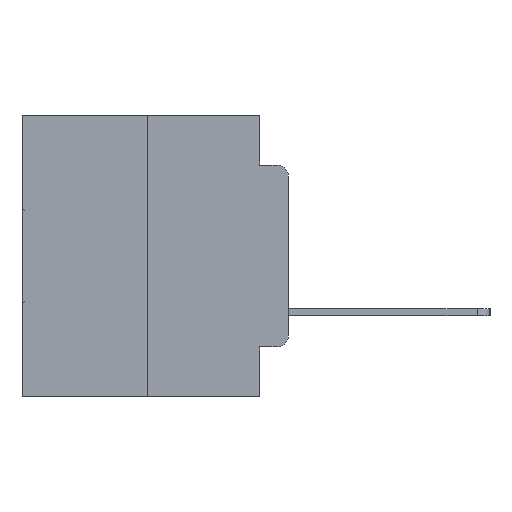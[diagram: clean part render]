
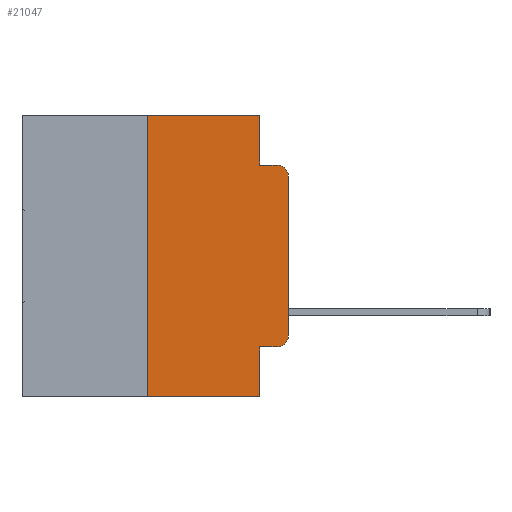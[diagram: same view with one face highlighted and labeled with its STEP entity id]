
A CAD part, left-side view. The second image highlights one B-rep face of the part: STEP entity #21047.
In plain terms, the highlighted planar face has unit normal (-1, 0, 0).
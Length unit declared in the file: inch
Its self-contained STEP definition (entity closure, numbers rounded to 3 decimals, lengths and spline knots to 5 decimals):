
#730 = LINE ( 'NONE', #3801, #25621 ) ;
#1275 = CARTESIAN_POINT ( 'NONE',  ( 0., 0.051, 0. ) ) ;
#1416 = LINE ( 'NONE', #19084, #6459 ) ;
#2512 = LINE ( 'NONE', #1275, #3318 ) ;
#3004 = AXIS2_PLACEMENT_3D ( 'NONE', #23975, #26347, #12099 ) ;
#3126 = DIRECTION ( 'NONE',  ( 0., 0., -1. ) ) ;
#3318 = VECTOR ( 'NONE', #15873, 39.37008 ) ;
#3801 = CARTESIAN_POINT ( 'NONE',  ( 0., 0.051, -0.0885 ) ) ;
#4295 = DIRECTION ( 'NONE',  ( 0., 0., 1. ) ) ;
#4416 = VECTOR ( 'NONE', #3126, 39.37008 ) ;
#5828 = VERTEX_POINT ( 'NONE', #13246 ) ;
#6107 = EDGE_LOOP ( 'NONE', ( #14253, #14192, #24177, #22808, #21876, #26127, #22690, #24151, #16340, #26494 ) ) ;
#6459 = VECTOR ( 'NONE', #7069, 39.37008 ) ;
#6887 = CARTESIAN_POINT ( 'NONE',  ( 0., 0.02, -0.0885 ) ) ;
#7069 = DIRECTION ( 'NONE',  ( 0., -1., 0. ) ) ;
#7168 = CARTESIAN_POINT ( 'NONE',  ( 0., 0.473, 0. ) ) ;
#7657 = CARTESIAN_POINT ( 'NONE',  ( 0., 0.051, -0.0885 ) ) ;
#7679 = CARTESIAN_POINT ( 'NONE',  ( 0., 0.02, -0.1085 ) ) ;
#8980 = DIRECTION ( 'NONE',  ( 0., 0., 1. ) ) ;
#9195 = EDGE_CURVE ( 'NONE', #5828, #19110, #17359, .T. ) ;
#9379 = EDGE_CURVE ( 'NONE', #13837, #19236, #24779, .T. ) ;
#9570 = DIRECTION ( 'NONE',  ( 0., -1., 0. ) ) ;
#9639 = PLANE ( 'NONE',  #3004 ) ;
#9650 = VERTEX_POINT ( 'NONE', #20642 ) ;
#10081 = DIRECTION ( 'NONE',  ( 0., 0., -1. ) ) ;
#10268 = VECTOR ( 'NONE', #8980, 39.37008 ) ;
#10321 = DIRECTION ( 'NONE',  ( -1., 0., 0. ) ) ;
#10883 = VECTOR ( 'NONE', #4295, 39.37008 ) ;
#11220 = CARTESIAN_POINT ( 'NONE',  ( 0., 0.051, 0. ) ) ;
#11739 = VECTOR ( 'NONE', #28634, 39.37008 ) ;
#12099 = DIRECTION ( 'NONE',  ( 0., 0., -1. ) ) ;
#12640 = EDGE_CURVE ( 'NONE', #15232, #13837, #1416, .T. ) ;
#13246 = CARTESIAN_POINT ( 'NONE',  ( 0., 0.25, -0.5 ) ) ;
#13837 = VERTEX_POINT ( 'NONE', #14783 ) ;
#14192 = ORIENTED_EDGE ( 'NONE', *, *, #25402, .T. ) ;
#14223 = EDGE_CURVE ( 'NONE', #15232, #19110, #2512, .T. ) ;
#14253 = ORIENTED_EDGE ( 'NONE', *, *, #26997, .T. ) ;
#14451 = CARTESIAN_POINT ( 'NONE',  ( 0., 0.473, -0.5 ) ) ;
#14783 = CARTESIAN_POINT ( 'NONE',  ( 0., 0.02, -0.4115 ) ) ;
#14862 = AXIS2_PLACEMENT_3D ( 'NONE', #7679, #24398, #10081 ) ;
#15232 = VERTEX_POINT ( 'NONE', #27882 ) ;
#15873 = DIRECTION ( 'NONE',  ( 0., 0., -1. ) ) ;
#16340 = ORIENTED_EDGE ( 'NONE', *, *, #12640, .T. ) ;
#16685 = LINE ( 'NONE', #23308, #10268 ) ;
#17145 = CARTESIAN_POINT ( 'NONE',  ( 0., 0., -0.3915 ) ) ;
#17173 = LINE ( 'NONE', #17552, #4416 ) ;
#17248 = LINE ( 'NONE', #18634, #10883 ) ;
#17359 = LINE ( 'NONE', #14451, #11739 ) ;
#17552 = CARTESIAN_POINT ( 'NONE',  ( 0., 0.051, 0. ) ) ;
#17777 = VERTEX_POINT ( 'NONE', #7657 ) ;
#18563 = LINE ( 'NONE', #7168, #30358 ) ;
#18634 = CARTESIAN_POINT ( 'NONE',  ( 0., 0., 0. ) ) ;
#18833 = CIRCLE ( 'NONE', #14862, 0.02 ) ;
#18992 = EDGE_CURVE ( 'NONE', #5828, #21230, #16685, .T. ) ;
#19084 = CARTESIAN_POINT ( 'NONE',  ( 0., 0.051, -0.4115 ) ) ;
#19110 = VERTEX_POINT ( 'NONE', #28426 ) ;
#19236 = VERTEX_POINT ( 'NONE', #17145 ) ;
#20588 = EDGE_CURVE ( 'NONE', #21505, #17777, #17173, .T. ) ;
#20642 = CARTESIAN_POINT ( 'NONE',  ( 0., 0., -0.1085 ) ) ;
#21047 = ADVANCED_FACE ( 'NONE', ( #22740 ), #9639, .F. ) ;
#21230 = VERTEX_POINT ( 'NONE', #26873 ) ;
#21505 = VERTEX_POINT ( 'NONE', #11220 ) ;
#21602 = VERTEX_POINT ( 'NONE', #6887 ) ;
#21839 = EDGE_CURVE ( 'NONE', #21230, #21505, #18563, .T. ) ;
#21876 = ORIENTED_EDGE ( 'NONE', *, *, #21839, .F. ) ;
#22206 = EDGE_CURVE ( 'NONE', #17777, #21602, #730, .T. ) ;
#22690 = ORIENTED_EDGE ( 'NONE', *, *, #9195, .T. ) ;
#22740 = FACE_OUTER_BOUND ( 'NONE', #6107, .T. ) ;
#22808 = ORIENTED_EDGE ( 'NONE', *, *, #20588, .F. ) ;
#22953 = DIRECTION ( 'NONE',  ( 0., -1., 0. ) ) ;
#23308 = CARTESIAN_POINT ( 'NONE',  ( 0., 0.25, 0. ) ) ;
#23975 = CARTESIAN_POINT ( 'NONE',  ( 0., 0.473, 0. ) ) ;
#24151 = ORIENTED_EDGE ( 'NONE', *, *, #14223, .F. ) ;
#24177 = ORIENTED_EDGE ( 'NONE', *, *, #22206, .F. ) ;
#24398 = DIRECTION ( 'NONE',  ( -1., 0., 0. ) ) ;
#24633 = CARTESIAN_POINT ( 'NONE',  ( 0., 0.02, -0.3915 ) ) ;
#24779 = CIRCLE ( 'NONE', #26037, 0.02 ) ;
#25402 = EDGE_CURVE ( 'NONE', #9650, #21602, #18833, .T. ) ;
#25621 = VECTOR ( 'NONE', #22953, 39.37008 ) ;
#26037 = AXIS2_PLACEMENT_3D ( 'NONE', #24633, #10321, #27025 ) ;
#26127 = ORIENTED_EDGE ( 'NONE', *, *, #18992, .F. ) ;
#26347 = DIRECTION ( 'NONE',  ( 1., 0., 0. ) ) ;
#26494 = ORIENTED_EDGE ( 'NONE', *, *, #9379, .T. ) ;
#26873 = CARTESIAN_POINT ( 'NONE',  ( 0., 0.25, 0. ) ) ;
#26997 = EDGE_CURVE ( 'NONE', #19236, #9650, #17248, .T. ) ;
#27025 = DIRECTION ( 'NONE',  ( 0., 0., -1. ) ) ;
#27882 = CARTESIAN_POINT ( 'NONE',  ( 0., 0.051, -0.4115 ) ) ;
#28426 = CARTESIAN_POINT ( 'NONE',  ( 0., 0.051, -0.5 ) ) ;
#28634 = DIRECTION ( 'NONE',  ( 0., -1., 0. ) ) ;
#30358 = VECTOR ( 'NONE', #9570, 39.37008 ) ;
